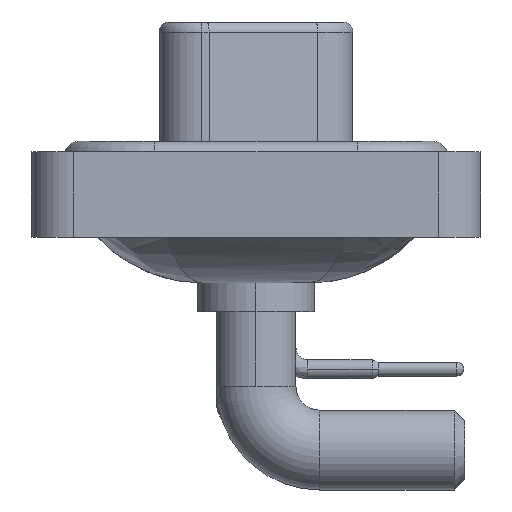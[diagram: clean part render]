
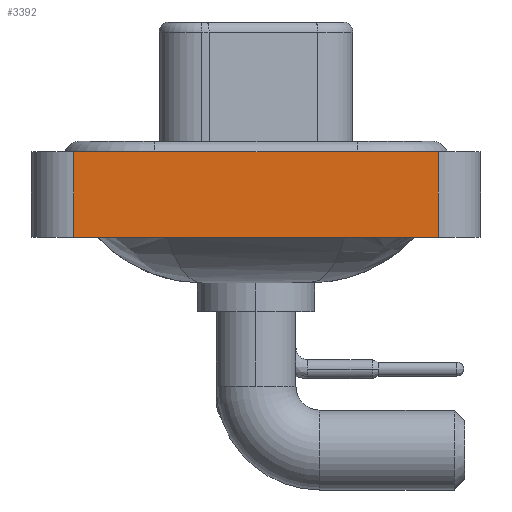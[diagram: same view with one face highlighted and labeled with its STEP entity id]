
A CAD part, left-side view. The second image highlights one B-rep face of the part: STEP entity #3392.
In plain terms, the highlighted planar face has unit normal (-1, 0, 0).
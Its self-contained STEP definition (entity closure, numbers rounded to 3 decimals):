
#155 = ORIENTED_EDGE ( 'NONE', *, *, #26404, .T. ) ;
#1014 = CARTESIAN_POINT ( 'NONE',  ( -7.35, 8.55, -3.6 ) ) ;
#1884 = EDGE_CURVE ( 'NONE', #23564, #19827, #16014, .T. ) ;
#1920 = DIRECTION ( 'NONE',  ( 0., 0., 1. ) ) ;
#1979 = CARTESIAN_POINT ( 'NONE',  ( -7.35, -8.55, -3.6 ) ) ;
#2275 = ORIENTED_EDGE ( 'NONE', *, *, #8828, .T. ) ;
#3392 = ADVANCED_FACE ( 'NONE', ( #8438 ), #18785, .T. ) ;
#4030 = LINE ( 'NONE', #8717, #4435 ) ;
#4302 = LINE ( 'NONE', #8324, #9659 ) ;
#4435 = VECTOR ( 'NONE', #16996, 1000. ) ;
#4438 = DIRECTION ( 'NONE',  ( 0., -1., 0. ) ) ;
#4868 = CARTESIAN_POINT ( 'NONE',  ( -7.35, 8.55, -3.6 ) ) ;
#6100 = ORIENTED_EDGE ( 'NONE', *, *, #1884, .F. ) ;
#6584 = CARTESIAN_POINT ( 'NONE',  ( -7.35, -8.55, 0.4 ) ) ;
#8060 = VECTOR ( 'NONE', #26434, 1000. ) ;
#8324 = CARTESIAN_POINT ( 'NONE',  ( -7.35, -8.55, -3.6 ) ) ;
#8416 = EDGE_LOOP ( 'NONE', ( #2275, #6100, #22874, #155 ) ) ;
#8438 = FACE_OUTER_BOUND ( 'NONE', #8416, .T. ) ;
#8701 = DIRECTION ( 'NONE',  ( -1., 0., 0. ) ) ;
#8717 = CARTESIAN_POINT ( 'NONE',  ( -7.35, -8.55, -3.6 ) ) ;
#8828 = EDGE_CURVE ( 'NONE', #22756, #19827, #4030, .T. ) ;
#9659 = VECTOR ( 'NONE', #4438, 1000. ) ;
#10505 = CARTESIAN_POINT ( 'NONE',  ( -7.35, -8.55, -3.6 ) ) ;
#16014 = LINE ( 'NONE', #16141, #19715 ) ;
#16141 = CARTESIAN_POINT ( 'NONE',  ( -7.35, -8.55, 0.4 ) ) ;
#16996 = DIRECTION ( 'NONE',  ( 0., 0., 1. ) ) ;
#17394 = VERTEX_POINT ( 'NONE', #4868 ) ;
#18372 = CARTESIAN_POINT ( 'NONE',  ( -7.35, 8.55, 0.4 ) ) ;
#18785 = PLANE ( 'NONE',  #22437 ) ;
#19715 = VECTOR ( 'NONE', #24311, 1000. ) ;
#19827 = VERTEX_POINT ( 'NONE', #6584 ) ;
#21423 = EDGE_CURVE ( 'NONE', #17394, #23564, #22174, .T. ) ;
#22174 = LINE ( 'NONE', #1014, #8060 ) ;
#22437 = AXIS2_PLACEMENT_3D ( 'NONE', #10505, #8701, #1920 ) ;
#22756 = VERTEX_POINT ( 'NONE', #1979 ) ;
#22874 = ORIENTED_EDGE ( 'NONE', *, *, #21423, .F. ) ;
#23564 = VERTEX_POINT ( 'NONE', #18372 ) ;
#24311 = DIRECTION ( 'NONE',  ( 0., -1., 0. ) ) ;
#26404 = EDGE_CURVE ( 'NONE', #17394, #22756, #4302, .T. ) ;
#26434 = DIRECTION ( 'NONE',  ( 0., 0., 1. ) ) ;
